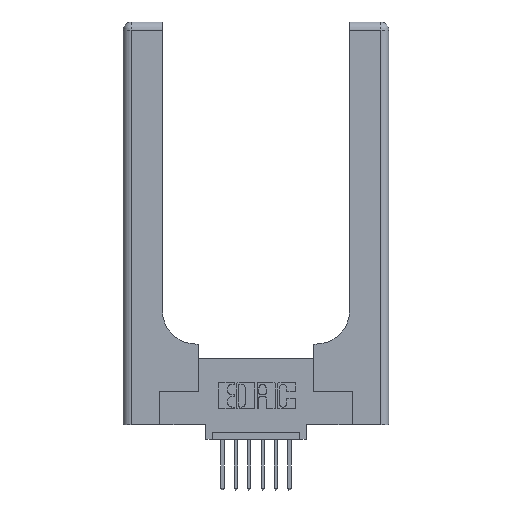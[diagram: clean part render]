
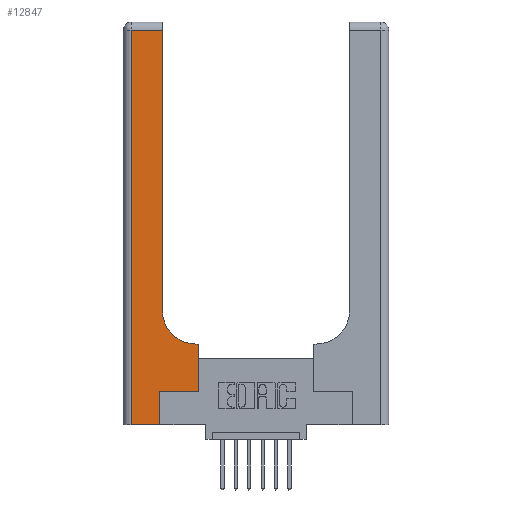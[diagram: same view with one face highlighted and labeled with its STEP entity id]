
A CAD part, top view. The second image highlights one B-rep face of the part: STEP entity #12847.
In plain terms, the highlighted planar face has unit normal (0, 0, 1).
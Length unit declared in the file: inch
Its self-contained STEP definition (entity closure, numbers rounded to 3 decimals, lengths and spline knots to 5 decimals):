
#289 = CARTESIAN_POINT ( 'NONE',  ( 0.2915, 2.94, 0.37 ) ) ;
#588 = AXIS2_PLACEMENT_3D ( 'NONE', #7289, #8591, #7341 ) ;
#1090 = EDGE_CURVE ( 'NONE', #6678, #1187, #11310, .T. ) ;
#1187 = VERTEX_POINT ( 'NONE', #5530 ) ;
#1261 = VECTOR ( 'NONE', #13333, 39.37008 ) ;
#1279 = LINE ( 'NONE', #13071, #13736 ) ;
#1365 = CARTESIAN_POINT ( 'NONE',  ( 0.06, 3., 0.37 ) ) ;
#1510 = EDGE_CURVE ( 'NONE', #9368, #14381, #4725, .T. ) ;
#1584 = CARTESIAN_POINT ( 'NONE',  ( 0.2915, 3., 0.37 ) ) ;
#1622 = ORIENTED_EDGE ( 'NONE', *, *, #1510, .T. ) ;
#2194 = LINE ( 'NONE', #12078, #3081 ) ;
#2214 = CARTESIAN_POINT ( 'NONE',  ( 0.5585, 0.25, 0.37 ) ) ;
#2346 = DIRECTION ( 'NONE',  ( -1., 0., 0. ) ) ;
#2658 = DIRECTION ( 'NONE',  ( 1., 0., 0. ) ) ;
#2753 = VECTOR ( 'NONE', #13341, 39.37008 ) ;
#3081 = VECTOR ( 'NONE', #12172, 39.37008 ) ;
#3242 = CARTESIAN_POINT ( 'NONE',  ( 0.06, 0., 0.37 ) ) ;
#3482 = DIRECTION ( 'NONE',  ( 0., -1., 0. ) ) ;
#3489 = VERTEX_POINT ( 'NONE', #13688 ) ;
#4094 = EDGE_CURVE ( 'NONE', #3489, #6678, #8046, .T. ) ;
#4191 = VERTEX_POINT ( 'NONE', #289 ) ;
#4256 = EDGE_LOOP ( 'NONE', ( #4929, #5526, #8192, #13797, #11098, #9183, #8631, #6900, #1622 ) ) ;
#4725 = CIRCLE ( 'NONE', #588, 0.25 ) ;
#4889 = LINE ( 'NONE', #7562, #2753 ) ;
#4929 = ORIENTED_EDGE ( 'NONE', *, *, #8304, .T. ) ;
#5526 = ORIENTED_EDGE ( 'NONE', *, *, #14607, .T. ) ;
#5530 = CARTESIAN_POINT ( 'NONE',  ( 0.269, 0., 0.37 ) ) ;
#5623 = VECTOR ( 'NONE', #10602, 39.37008 ) ;
#5684 = DIRECTION ( 'NONE',  ( 0., 0., -1. ) ) ;
#6678 = VERTEX_POINT ( 'NONE', #3242 ) ;
#6900 = ORIENTED_EDGE ( 'NONE', *, *, #13301, .T. ) ;
#7289 = CARTESIAN_POINT ( 'NONE',  ( 0.5415, 0.85, 0.37 ) ) ;
#7341 = DIRECTION ( 'NONE',  ( 1., 0., 0. ) ) ;
#7562 = CARTESIAN_POINT ( 'NONE',  ( 0.269, 0., 0.37 ) ) ;
#7911 = CARTESIAN_POINT ( 'NONE',  ( 0., 3., 0.37 ) ) ;
#8032 = LINE ( 'NONE', #2214, #1261 ) ;
#8046 = LINE ( 'NONE', #1365, #10720 ) ;
#8125 = CARTESIAN_POINT ( 'NONE',  ( 0.5585, 0.25, 0.37 ) ) ;
#8192 = ORIENTED_EDGE ( 'NONE', *, *, #4094, .T. ) ;
#8262 = DIRECTION ( 'NONE',  ( -1., 0., 0. ) ) ;
#8304 = EDGE_CURVE ( 'NONE', #14381, #4191, #14323, .T. ) ;
#8450 = CARTESIAN_POINT ( 'NONE',  ( 0., 0., 0.37 ) ) ;
#8472 = DIRECTION ( 'NONE',  ( 1., 0., 0. ) ) ;
#8491 = CARTESIAN_POINT ( 'NONE',  ( 0.5415, 0.6, 0.37 ) ) ;
#8534 = VERTEX_POINT ( 'NONE', #8125 ) ;
#8566 = CARTESIAN_POINT ( 'NONE',  ( 0.5585, 0.6, 0.37 ) ) ;
#8591 = DIRECTION ( 'NONE',  ( 0., 0., -1. ) ) ;
#8631 = ORIENTED_EDGE ( 'NONE', *, *, #12818, .T. ) ;
#8707 = VERTEX_POINT ( 'NONE', #8566 ) ;
#8830 = VECTOR ( 'NONE', #2658, 39.37008 ) ;
#8928 = EDGE_CURVE ( 'NONE', #1187, #14558, #4889, .T. ) ;
#9183 = ORIENTED_EDGE ( 'NONE', *, *, #9983, .T. ) ;
#9368 = VERTEX_POINT ( 'NONE', #8491 ) ;
#9983 = EDGE_CURVE ( 'NONE', #14558, #8534, #1279, .T. ) ;
#10043 = CARTESIAN_POINT ( 'NONE',  ( 0.2915, 0.85, 0.37 ) ) ;
#10267 = PLANE ( 'NONE',  #11563 ) ;
#10602 = DIRECTION ( 'NONE',  ( 0., 1., 0. ) ) ;
#10720 = VECTOR ( 'NONE', #3482, 39.37008 ) ;
#11033 = LINE ( 'NONE', #12495, #12793 ) ;
#11098 = ORIENTED_EDGE ( 'NONE', *, *, #8928, .T. ) ;
#11310 = LINE ( 'NONE', #8450, #8830 ) ;
#11563 = AXIS2_PLACEMENT_3D ( 'NONE', #7911, #5684, #2346 ) ;
#12078 = CARTESIAN_POINT ( 'NONE',  ( 0.2915, 0.6, 0.37 ) ) ;
#12172 = DIRECTION ( 'NONE',  ( -1., 0., 0. ) ) ;
#12495 = CARTESIAN_POINT ( 'NONE',  ( 0., 2.94, 0.37 ) ) ;
#12659 = FACE_OUTER_BOUND ( 'NONE', #4256, .T. ) ;
#12793 = VECTOR ( 'NONE', #8262, 39.37008 ) ;
#12818 = EDGE_CURVE ( 'NONE', #8534, #8707, #8032, .T. ) ;
#12847 = ADVANCED_FACE ( 'NONE', ( #12659 ), #10267, .F. ) ;
#13071 = CARTESIAN_POINT ( 'NONE',  ( 0.269, 0.25, 0.37 ) ) ;
#13301 = EDGE_CURVE ( 'NONE', #8707, #9368, #2194, .T. ) ;
#13333 = DIRECTION ( 'NONE',  ( 0., 1., 0. ) ) ;
#13341 = DIRECTION ( 'NONE',  ( 0., 1., 0. ) ) ;
#13549 = CARTESIAN_POINT ( 'NONE',  ( 0.269, 0.25, 0.37 ) ) ;
#13688 = CARTESIAN_POINT ( 'NONE',  ( 0.06, 2.94, 0.37 ) ) ;
#13736 = VECTOR ( 'NONE', #8472, 39.37008 ) ;
#13797 = ORIENTED_EDGE ( 'NONE', *, *, #1090, .T. ) ;
#14323 = LINE ( 'NONE', #1584, #5623 ) ;
#14381 = VERTEX_POINT ( 'NONE', #10043 ) ;
#14558 = VERTEX_POINT ( 'NONE', #13549 ) ;
#14607 = EDGE_CURVE ( 'NONE', #4191, #3489, #11033, .T. ) ;
